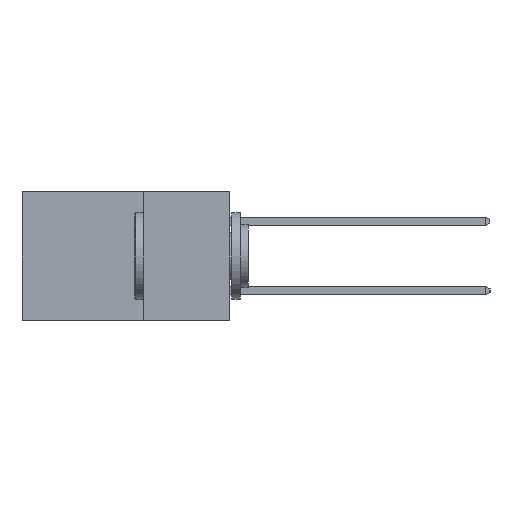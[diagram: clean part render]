
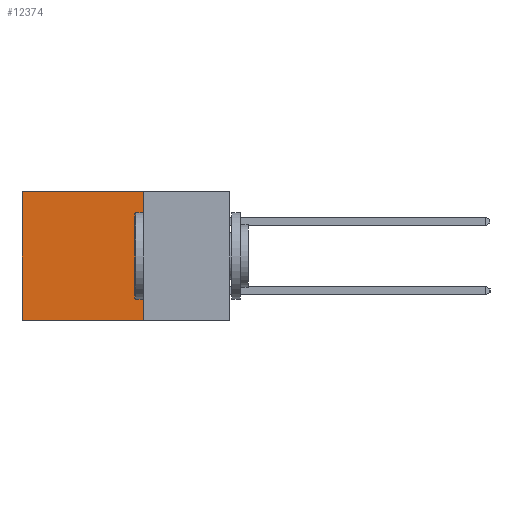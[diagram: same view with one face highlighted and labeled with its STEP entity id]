
A CAD part, left-side view. The second image highlights one B-rep face of the part: STEP entity #12374.
In plain terms, the highlighted planar face has unit normal (-1, 0, 0).
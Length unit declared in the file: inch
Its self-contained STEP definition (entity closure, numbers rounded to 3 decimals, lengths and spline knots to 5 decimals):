
#22 = DIRECTION ( 'NONE',  ( 1., 0., 0. ) ) ;
#287 = VECTOR ( 'NONE', #946, 39.37008 ) ;
#716 = LINE ( 'NONE', #4803, #287 ) ;
#946 = DIRECTION ( 'NONE',  ( 0., 1., 0. ) ) ;
#1132 = ORIENTED_EDGE ( 'NONE', *, *, #1147, .F. ) ;
#1147 = EDGE_CURVE ( 'NONE', #4020, #4147, #5548, .T. ) ;
#1292 = DIRECTION ( 'NONE',  ( 0., 1., 0. ) ) ;
#1962 = CARTESIAN_POINT ( 'NONE',  ( 0.2615, 0.6, -0.37 ) ) ;
#2669 = EDGE_CURVE ( 'NONE', #4020, #8354, #716, .T. ) ;
#3026 = CARTESIAN_POINT ( 'NONE',  ( 0.2615, 0.25, -0.37 ) ) ;
#3392 = VERTEX_POINT ( 'NONE', #1962 ) ;
#3902 = CARTESIAN_POINT ( 'NONE',  ( 0.2615, 0.25, -0.37 ) ) ;
#4020 = VERTEX_POINT ( 'NONE', #7193 ) ;
#4083 = CARTESIAN_POINT ( 'NONE',  ( 0.2615, 0.6, -0.37 ) ) ;
#4147 = VERTEX_POINT ( 'NONE', #3026 ) ;
#4803 = CARTESIAN_POINT ( 'NONE',  ( 0.2615, 0.25, 0. ) ) ;
#5156 = DIRECTION ( 'NONE',  ( 0., 0., -1. ) ) ;
#5548 = LINE ( 'NONE', #12006, #15118 ) ;
#5597 = CARTESIAN_POINT ( 'NONE',  ( 0.2615, 0.6, 0. ) ) ;
#6602 = EDGE_LOOP ( 'NONE', ( #11163, #10858, #1132, #7937 ) ) ;
#7193 = CARTESIAN_POINT ( 'NONE',  ( 0.2615, 0.25, 0. ) ) ;
#7937 = ORIENTED_EDGE ( 'NONE', *, *, #2669, .T. ) ;
#7967 = PLANE ( 'NONE',  #14821 ) ;
#8354 = VERTEX_POINT ( 'NONE', #5597 ) ;
#9183 = VECTOR ( 'NONE', #13272, 39.37008 ) ;
#9291 = DIRECTION ( 'NONE',  ( 0., 0., -1. ) ) ;
#9596 = EDGE_CURVE ( 'NONE', #4147, #3392, #14522, .T. ) ;
#10858 = ORIENTED_EDGE ( 'NONE', *, *, #9596, .F. ) ;
#11108 = VECTOR ( 'NONE', #1292, 39.37008 ) ;
#11163 = ORIENTED_EDGE ( 'NONE', *, *, #16852, .T. ) ;
#12006 = CARTESIAN_POINT ( 'NONE',  ( 0.2615, 0.25, -0.37 ) ) ;
#12374 = ADVANCED_FACE ( 'NONE', ( #14591 ), #7967, .F. ) ;
#13272 = DIRECTION ( 'NONE',  ( 0., 0., -1. ) ) ;
#14522 = LINE ( 'NONE', #3902, #11108 ) ;
#14591 = FACE_OUTER_BOUND ( 'NONE', #6602, .T. ) ;
#14821 = AXIS2_PLACEMENT_3D ( 'NONE', #15705, #22, #9291 ) ;
#15118 = VECTOR ( 'NONE', #5156, 39.37008 ) ;
#15705 = CARTESIAN_POINT ( 'NONE',  ( 0.2615, 0.25, -0.37 ) ) ;
#16046 = LINE ( 'NONE', #4083, #9183 ) ;
#16852 = EDGE_CURVE ( 'NONE', #8354, #3392, #16046, .T. ) ;
